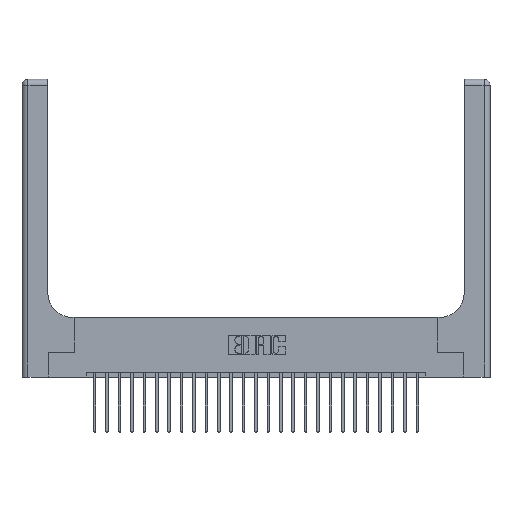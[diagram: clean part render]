
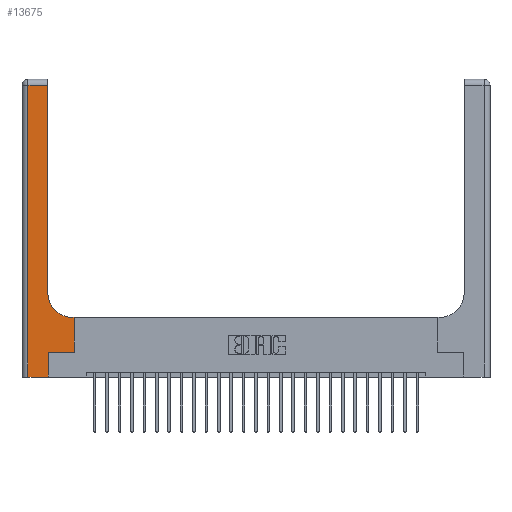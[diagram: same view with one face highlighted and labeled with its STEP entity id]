
A CAD part, top view. The second image highlights one B-rep face of the part: STEP entity #13675.
In plain terms, the highlighted planar face has unit normal (0, 0, 1).
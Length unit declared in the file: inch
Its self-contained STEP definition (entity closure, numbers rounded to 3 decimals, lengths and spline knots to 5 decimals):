
#144 = VECTOR ( 'NONE', #4378, 39.37008 ) ;
#1152 = LINE ( 'NONE', #11531, #1767 ) ;
#1587 = VERTEX_POINT ( 'NONE', #14994 ) ;
#1767 = VECTOR ( 'NONE', #9771, 39.37008 ) ;
#1857 = VERTEX_POINT ( 'NONE', #17643 ) ;
#2418 = ORIENTED_EDGE ( 'NONE', *, *, #18759, .T. ) ;
#2576 = CARTESIAN_POINT ( 'NONE',  ( 0.528, 0.25, 0.37 ) ) ;
#2866 = CARTESIAN_POINT ( 'NONE',  ( 0., 3., 0.37 ) ) ;
#3864 = CIRCLE ( 'NONE', #10219, 0.25 ) ;
#4179 = DIRECTION ( 'NONE',  ( 1., 0., 0. ) ) ;
#4378 = DIRECTION ( 'NONE',  ( 0., 1., 0. ) ) ;
#4406 = CARTESIAN_POINT ( 'NONE',  ( 0.265, 0., 0.37 ) ) ;
#4460 = DIRECTION ( 'NONE',  ( 1., 0., 0. ) ) ;
#4534 = EDGE_CURVE ( 'NONE', #1587, #1857, #15464, .T. ) ;
#4795 = VECTOR ( 'NONE', #24699, 39.37008 ) ;
#5055 = VERTEX_POINT ( 'NONE', #22410 ) ;
#5399 = ORIENTED_EDGE ( 'NONE', *, *, #7859, .T. ) ;
#6717 = AXIS2_PLACEMENT_3D ( 'NONE', #2866, #9543, #7634 ) ;
#6969 = LINE ( 'NONE', #23529, #14178 ) ;
#7025 = CARTESIAN_POINT ( 'NONE',  ( 0.265, 0.25, 0.37 ) ) ;
#7354 = LINE ( 'NONE', #9070, #13347 ) ;
#7484 = DIRECTION ( 'NONE',  ( -1., 0., 0. ) ) ;
#7634 = DIRECTION ( 'NONE',  ( -1., 0., 0. ) ) ;
#7859 = EDGE_CURVE ( 'NONE', #19176, #5055, #12384, .T. ) ;
#7904 = CARTESIAN_POINT ( 'NONE',  ( 0., 2.94, 0.37 ) ) ;
#8149 = CARTESIAN_POINT ( 'NONE',  ( 0.06, 2.94, 0.37 ) ) ;
#8226 = CARTESIAN_POINT ( 'NONE',  ( 0.51, 0.85, 0.37 ) ) ;
#9070 = CARTESIAN_POINT ( 'NONE',  ( 0., 0., 0.37 ) ) ;
#9288 = CARTESIAN_POINT ( 'NONE',  ( 0.06, 3., 0.37 ) ) ;
#9342 = VERTEX_POINT ( 'NONE', #11115 ) ;
#9382 = EDGE_CURVE ( 'NONE', #23536, #20058, #1152, .T. ) ;
#9514 = DIRECTION ( 'NONE',  ( -1., 0., 0. ) ) ;
#9543 = DIRECTION ( 'NONE',  ( 0., 0., -1. ) ) ;
#9771 = DIRECTION ( 'NONE',  ( 0., 1., 0. ) ) ;
#9799 = EDGE_CURVE ( 'NONE', #1857, #9342, #21551, .T. ) ;
#10219 = AXIS2_PLACEMENT_3D ( 'NONE', #8226, #21463, #4460 ) ;
#10434 = EDGE_CURVE ( 'NONE', #9342, #23536, #3864, .T. ) ;
#10520 = DIRECTION ( 'NONE',  ( 1., 0., 0. ) ) ;
#11115 = CARTESIAN_POINT ( 'NONE',  ( 0.51, 0.6, 0.37 ) ) ;
#11474 = ORIENTED_EDGE ( 'NONE', *, *, #10434, .T. ) ;
#11531 = CARTESIAN_POINT ( 'NONE',  ( 0.26, 3., 0.37 ) ) ;
#12309 = EDGE_LOOP ( 'NONE', ( #24567, #23763, #5399, #2418, #22391, #22320, #21785, #13230, #11474 ) ) ;
#12384 = LINE ( 'NONE', #9288, #14186 ) ;
#12618 = VECTOR ( 'NONE', #7484, 39.37008 ) ;
#13230 = ORIENTED_EDGE ( 'NONE', *, *, #9799, .T. ) ;
#13347 = VECTOR ( 'NONE', #10520, 39.37008 ) ;
#13463 = EDGE_CURVE ( 'NONE', #19407, #1587, #6969, .T. ) ;
#13467 = CARTESIAN_POINT ( 'NONE',  ( 0.265, 0., 0.37 ) ) ;
#13675 = ADVANCED_FACE ( 'NONE', ( #17132 ), #21979, .F. ) ;
#14178 = VECTOR ( 'NONE', #4179, 39.37008 ) ;
#14186 = VECTOR ( 'NONE', #24629, 39.37008 ) ;
#14994 = CARTESIAN_POINT ( 'NONE',  ( 0.528, 0.25, 0.37 ) ) ;
#15125 = EDGE_CURVE ( 'NONE', #20023, #19407, #18870, .T. ) ;
#15196 = VECTOR ( 'NONE', #9514, 39.37008 ) ;
#15464 = LINE ( 'NONE', #2576, #144 ) ;
#17132 = FACE_OUTER_BOUND ( 'NONE', #12309, .T. ) ;
#17643 = CARTESIAN_POINT ( 'NONE',  ( 0.528, 0.6, 0.37 ) ) ;
#18062 = CARTESIAN_POINT ( 'NONE',  ( 0.26, 0.85, 0.37 ) ) ;
#18759 = EDGE_CURVE ( 'NONE', #5055, #20023, #7354, .T. ) ;
#18870 = LINE ( 'NONE', #13467, #4795 ) ;
#19176 = VERTEX_POINT ( 'NONE', #8149 ) ;
#19407 = VERTEX_POINT ( 'NONE', #7025 ) ;
#20023 = VERTEX_POINT ( 'NONE', #4406 ) ;
#20058 = VERTEX_POINT ( 'NONE', #21806 ) ;
#21463 = DIRECTION ( 'NONE',  ( 0., 0., -1. ) ) ;
#21551 = LINE ( 'NONE', #22801, #12618 ) ;
#21785 = ORIENTED_EDGE ( 'NONE', *, *, #4534, .T. ) ;
#21806 = CARTESIAN_POINT ( 'NONE',  ( 0.26, 2.94, 0.37 ) ) ;
#21979 = PLANE ( 'NONE',  #6717 ) ;
#22320 = ORIENTED_EDGE ( 'NONE', *, *, #13463, .T. ) ;
#22391 = ORIENTED_EDGE ( 'NONE', *, *, #15125, .T. ) ;
#22410 = CARTESIAN_POINT ( 'NONE',  ( 0.06, 0., 0.37 ) ) ;
#22679 = LINE ( 'NONE', #7904, #15196 ) ;
#22801 = CARTESIAN_POINT ( 'NONE',  ( 0.26, 0.6, 0.37 ) ) ;
#22807 = EDGE_CURVE ( 'NONE', #20058, #19176, #22679, .T. ) ;
#23529 = CARTESIAN_POINT ( 'NONE',  ( 0.265, 0.25, 0.37 ) ) ;
#23536 = VERTEX_POINT ( 'NONE', #18062 ) ;
#23763 = ORIENTED_EDGE ( 'NONE', *, *, #22807, .T. ) ;
#24567 = ORIENTED_EDGE ( 'NONE', *, *, #9382, .T. ) ;
#24629 = DIRECTION ( 'NONE',  ( 0., -1., 0. ) ) ;
#24699 = DIRECTION ( 'NONE',  ( 0., 1., 0. ) ) ;
